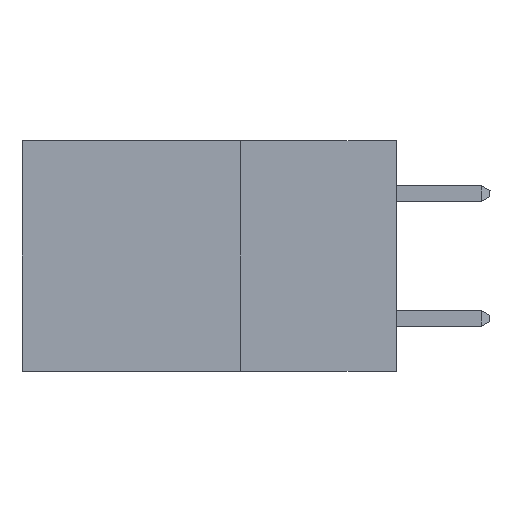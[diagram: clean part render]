
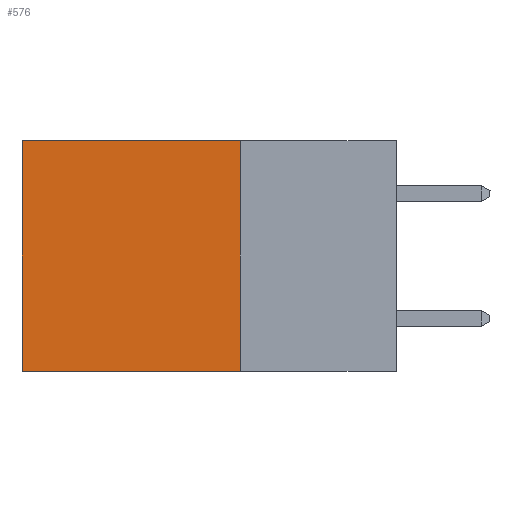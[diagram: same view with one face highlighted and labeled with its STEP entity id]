
A CAD part, left-side view. The second image highlights one B-rep face of the part: STEP entity #576.
In plain terms, the highlighted planar face has unit normal (-1, 0, 0).
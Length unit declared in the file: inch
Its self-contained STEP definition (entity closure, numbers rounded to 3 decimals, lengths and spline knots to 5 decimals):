
#159 = VERTEX_POINT ( 'NONE', #10492 ) ;
#451 = VERTEX_POINT ( 'NONE', #2873 ) ;
#576 = ADVANCED_FACE ( 'NONE', ( #8202 ), #5742, .F. ) ;
#829 = LINE ( 'NONE', #6161, #4965 ) ;
#864 = AXIS2_PLACEMENT_3D ( 'NONE', #7220, #7037, #6719 ) ;
#1037 = VECTOR ( 'NONE', #10309, 39.37008 ) ;
#1172 = VECTOR ( 'NONE', #2735, 39.37008 ) ;
#2537 = CARTESIAN_POINT ( 'NONE',  ( 0.298, 0.25, 0. ) ) ;
#2704 = VERTEX_POINT ( 'NONE', #10162 ) ;
#2735 = DIRECTION ( 'NONE',  ( 0., 1., 0. ) ) ;
#2873 = CARTESIAN_POINT ( 'NONE',  ( 0.298, 0.25, -0.37 ) ) ;
#2999 = CARTESIAN_POINT ( 'NONE',  ( 0.298, 0.25, 0. ) ) ;
#3002 = LINE ( 'NONE', #10321, #1037 ) ;
#3266 = EDGE_CURVE ( 'NONE', #159, #7021, #3002, .T. ) ;
#3448 = EDGE_CURVE ( 'NONE', #2704, #159, #7467, .T. ) ;
#4189 = ORIENTED_EDGE ( 'NONE', *, *, #3266, .T. ) ;
#4965 = VECTOR ( 'NONE', #6628, 39.37008 ) ;
#5168 = ORIENTED_EDGE ( 'NONE', *, *, #5793, .F. ) ;
#5280 = ORIENTED_EDGE ( 'NONE', *, *, #10214, .F. ) ;
#5425 = ORIENTED_EDGE ( 'NONE', *, *, #3448, .T. ) ;
#5742 = PLANE ( 'NONE',  #864 ) ;
#5793 = EDGE_CURVE ( 'NONE', #451, #7021, #829, .T. ) ;
#6161 = CARTESIAN_POINT ( 'NONE',  ( 0.298, 0.25, -0.37 ) ) ;
#6628 = DIRECTION ( 'NONE',  ( 0., 1., 0. ) ) ;
#6719 = DIRECTION ( 'NONE',  ( 0., 0., -1. ) ) ;
#6967 = EDGE_LOOP ( 'NONE', ( #4189, #5168, #5280, #5425 ) ) ;
#7021 = VERTEX_POINT ( 'NONE', #9546 ) ;
#7037 = DIRECTION ( 'NONE',  ( 1., 0., 0. ) ) ;
#7220 = CARTESIAN_POINT ( 'NONE',  ( 0.298, 0.25, 0. ) ) ;
#7467 = LINE ( 'NONE', #2537, #1172 ) ;
#7719 = VECTOR ( 'NONE', #7935, 39.37008 ) ;
#7935 = DIRECTION ( 'NONE',  ( 0., 0., -1. ) ) ;
#8202 = FACE_OUTER_BOUND ( 'NONE', #6967, .T. ) ;
#9546 = CARTESIAN_POINT ( 'NONE',  ( 0.298, 0.6, -0.37 ) ) ;
#9856 = LINE ( 'NONE', #2999, #7719 ) ;
#10162 = CARTESIAN_POINT ( 'NONE',  ( 0.298, 0.25, 0. ) ) ;
#10214 = EDGE_CURVE ( 'NONE', #2704, #451, #9856, .T. ) ;
#10309 = DIRECTION ( 'NONE',  ( 0., 0., -1. ) ) ;
#10321 = CARTESIAN_POINT ( 'NONE',  ( 0.298, 0.6, 0. ) ) ;
#10492 = CARTESIAN_POINT ( 'NONE',  ( 0.298, 0.6, 0. ) ) ;
